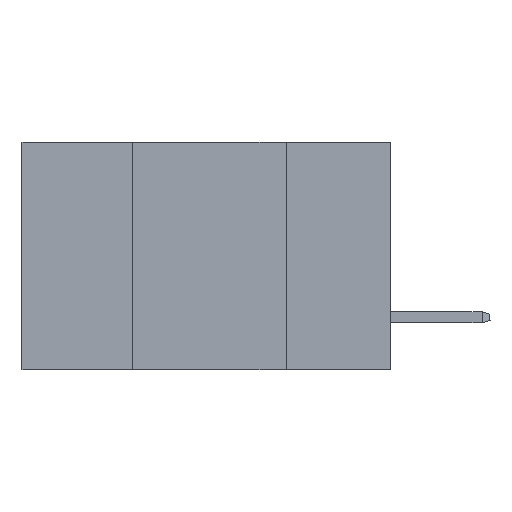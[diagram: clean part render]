
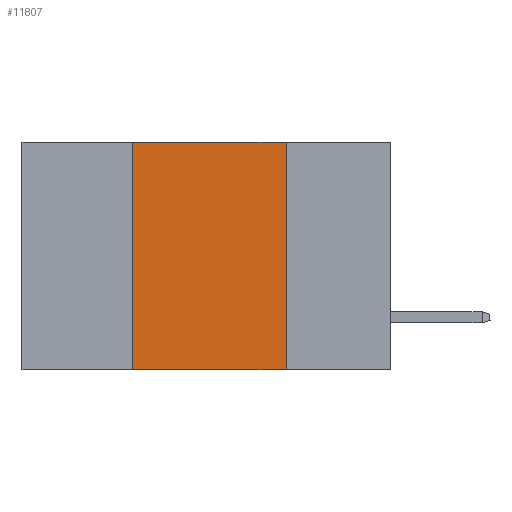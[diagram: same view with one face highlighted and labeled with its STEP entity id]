
A CAD part, left-side view. The second image highlights one B-rep face of the part: STEP entity #11807.
In plain terms, the highlighted planar face has unit normal (-1, 0, 0).
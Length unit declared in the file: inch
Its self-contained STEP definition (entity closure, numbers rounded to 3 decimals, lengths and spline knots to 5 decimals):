
#645 = DIRECTION ( 'NONE',  ( 0., 0., -1. ) ) ;
#882 = EDGE_CURVE ( 'NONE', #8221, #6164, #5136, .T. ) ;
#1518 = ORIENTED_EDGE ( 'NONE', *, *, #882, .F. ) ;
#1649 = CARTESIAN_POINT ( 'NONE',  ( 0., 0.6, -0.37 ) ) ;
#1784 = EDGE_LOOP ( 'NONE', ( #9128, #2675, #1518, #11877 ) ) ;
#1862 = LINE ( 'NONE', #4859, #7104 ) ;
#1900 = VECTOR ( 'NONE', #3464, 39.37008 ) ;
#1947 = DIRECTION ( 'NONE',  ( 0., -1., 0. ) ) ;
#2393 = VECTOR ( 'NONE', #9083, 39.37008 ) ;
#2495 = CARTESIAN_POINT ( 'NONE',  ( 0., 0.42, 0. ) ) ;
#2521 = LINE ( 'NONE', #9093, #7618 ) ;
#2675 = ORIENTED_EDGE ( 'NONE', *, *, #3165, .F. ) ;
#2745 = VERTEX_POINT ( 'NONE', #8657 ) ;
#3165 = EDGE_CURVE ( 'NONE', #6164, #2745, #1862, .T. ) ;
#3256 = CARTESIAN_POINT ( 'NONE',  ( 0., 0.42, -0.37 ) ) ;
#3464 = DIRECTION ( 'NONE',  ( 0., 0., 1. ) ) ;
#4167 = LINE ( 'NONE', #1649, #2393 ) ;
#4711 = EDGE_CURVE ( 'NONE', #8221, #11045, #4167, .T. ) ;
#4859 = CARTESIAN_POINT ( 'NONE',  ( 0., 0.6, 0. ) ) ;
#5136 = LINE ( 'NONE', #5384, #1900 ) ;
#5384 = CARTESIAN_POINT ( 'NONE',  ( 0., 0.42, 0. ) ) ;
#5398 = CARTESIAN_POINT ( 'NONE',  ( 0., 0.17, -0.37 ) ) ;
#5960 = DIRECTION ( 'NONE',  ( 0., 0., -1. ) ) ;
#6040 = DIRECTION ( 'NONE',  ( 1., 0., 0. ) ) ;
#6164 = VERTEX_POINT ( 'NONE', #2495 ) ;
#6458 = EDGE_CURVE ( 'NONE', #2745, #11045, #2521, .T. ) ;
#7104 = VECTOR ( 'NONE', #1947, 39.37008 ) ;
#7618 = VECTOR ( 'NONE', #645, 39.37008 ) ;
#8221 = VERTEX_POINT ( 'NONE', #3256 ) ;
#8572 = AXIS2_PLACEMENT_3D ( 'NONE', #9633, #6040, #5960 ) ;
#8657 = CARTESIAN_POINT ( 'NONE',  ( 0., 0.17, 0. ) ) ;
#9083 = DIRECTION ( 'NONE',  ( 0., -1., 0. ) ) ;
#9093 = CARTESIAN_POINT ( 'NONE',  ( 0., 0.17, 0. ) ) ;
#9128 = ORIENTED_EDGE ( 'NONE', *, *, #6458, .F. ) ;
#9633 = CARTESIAN_POINT ( 'NONE',  ( 0., 0.6, 0. ) ) ;
#9713 = PLANE ( 'NONE',  #8572 ) ;
#10316 = FACE_OUTER_BOUND ( 'NONE', #1784, .T. ) ;
#11045 = VERTEX_POINT ( 'NONE', #5398 ) ;
#11807 = ADVANCED_FACE ( 'NONE', ( #10316 ), #9713, .F. ) ;
#11877 = ORIENTED_EDGE ( 'NONE', *, *, #4711, .T. ) ;
